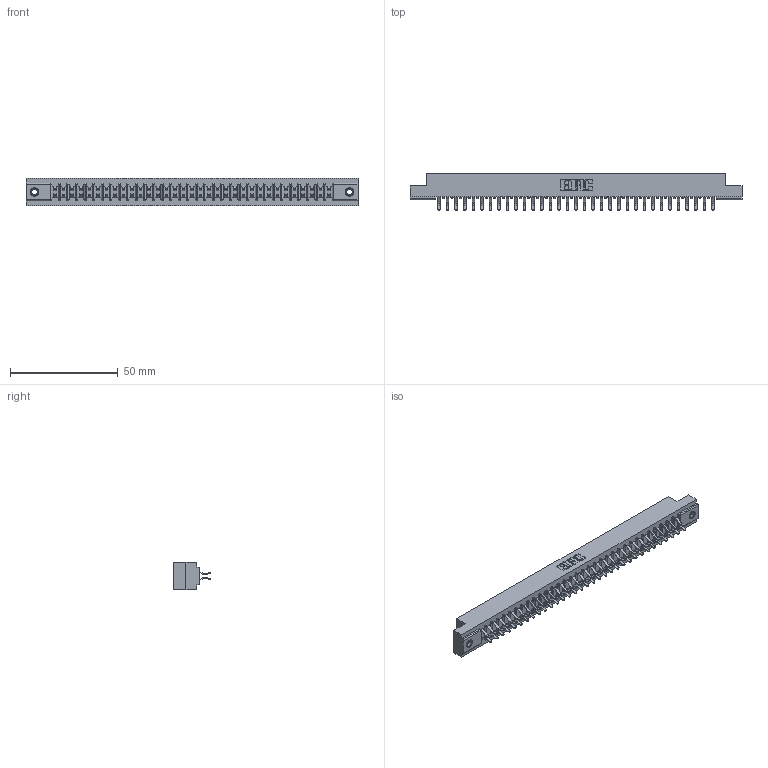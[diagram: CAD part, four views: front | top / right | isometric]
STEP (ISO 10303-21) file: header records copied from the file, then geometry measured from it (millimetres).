
FILE_DESCRIPTION (( 'STEP AP203' ), '1' );
FILE_NAME ('307-066-456-207.STEP', '2020-09-30T19:59:13', ( '' ), ( '' ), 'SwSTEP 2.0', 'SolidWorks 2020', '' );
FILE_SCHEMA (( 'CONFIG_CONTROL_DESIGN' ));
Length unit declared in the file: inch
Products named in the file (4): 345-250-001_345-250-005-103; 307-290-001_556; 307 Part_.156 Dia Mounting Holes; 307-066-456-207
Assembly tree (69 placements, depth 2):
  307-066-456-207
    307 Part_.156 Dia Mounting Holes
    307-290-001_556  x66
    345-250-001_345-250-005-103  x2
Bounding box: 153.77 x 16.97 x 12.7 mm (x, y, z)
Volume: 16262.5 mm3; surface area: 19575.9 mm2
Topology: 69 solids, 69 shells, 3512 faces, 9831 edges, 6366 vertices
Faces by surface type: plane 2280, cylinder 1148, sphere 68, cone 12, torus 4
Entity records: 31745 total; most frequent: CARTESIAN_POINT 5180, ORIENTED_EDGE 5126, DIRECTION 5087, EDGE_CURVE 2563, LINE 1961, VECTOR 1961, VERTEX_POINT 1656, AXIS2_PLACEMENT_3D 1563
